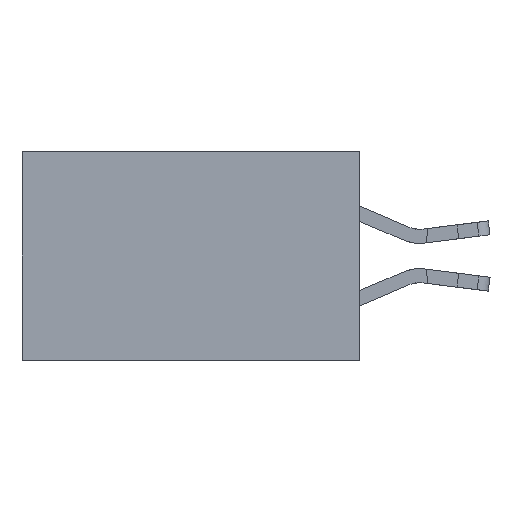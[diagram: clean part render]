
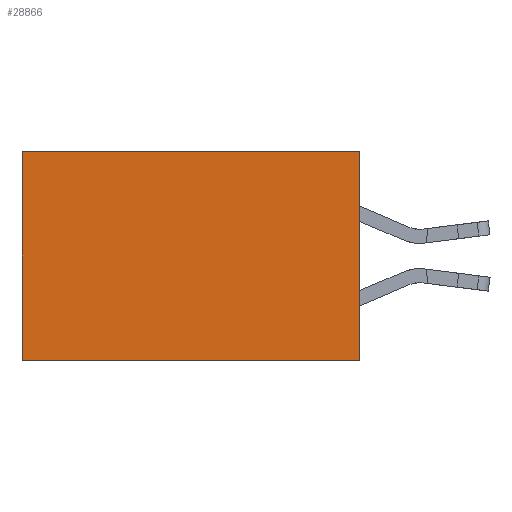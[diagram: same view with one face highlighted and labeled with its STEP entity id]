
A CAD part, left-side view. The second image highlights one B-rep face of the part: STEP entity #28866.
In plain terms, the highlighted planar face has unit normal (-1, 0, 0).
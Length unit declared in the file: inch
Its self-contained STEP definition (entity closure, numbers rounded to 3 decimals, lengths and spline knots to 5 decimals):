
#1132 = PLANE ( 'NONE',  #10331 ) ;
#1287 = CARTESIAN_POINT ( 'NONE',  ( 0.2875, 0., 0. ) ) ;
#1408 = EDGE_CURVE ( 'NONE', #7992, #14091, #3593, .T. ) ;
#1514 = CARTESIAN_POINT ( 'NONE',  ( 0.2875, 0.6, 0. ) ) ;
#1757 = CARTESIAN_POINT ( 'NONE',  ( 0.2875, 0., -0.37 ) ) ;
#1808 = DIRECTION ( 'NONE',  ( 0., 0., -1. ) ) ;
#2328 = LINE ( 'NONE', #1287, #7299 ) ;
#3593 = LINE ( 'NONE', #5527, #18698 ) ;
#3740 = DIRECTION ( 'NONE',  ( 0., 0., -1. ) ) ;
#5527 = CARTESIAN_POINT ( 'NONE',  ( 0.2875, 0., 0. ) ) ;
#5726 = DIRECTION ( 'NONE',  ( 0., 1., 0. ) ) ;
#5927 = ORIENTED_EDGE ( 'NONE', *, *, #18400, .F. ) ;
#7299 = VECTOR ( 'NONE', #3740, 39.37008 ) ;
#7992 = VERTEX_POINT ( 'NONE', #8667 ) ;
#8015 = DIRECTION ( 'NONE',  ( 1., 0., 0. ) ) ;
#8667 = CARTESIAN_POINT ( 'NONE',  ( 0.2875, 0., 0. ) ) ;
#9554 = CARTESIAN_POINT ( 'NONE',  ( 0.2875, 0., -0.37 ) ) ;
#10331 = AXIS2_PLACEMENT_3D ( 'NONE', #26104, #8015, #25819 ) ;
#11469 = EDGE_LOOP ( 'NONE', ( #28283, #20543, #5927, #12987 ) ) ;
#11932 = LINE ( 'NONE', #1514, #24265 ) ;
#12057 = EDGE_CURVE ( 'NONE', #25491, #14859, #18609, .T. ) ;
#12987 = ORIENTED_EDGE ( 'NONE', *, *, #1408, .T. ) ;
#13272 = CARTESIAN_POINT ( 'NONE',  ( 0.2875, 0.6, 0. ) ) ;
#14091 = VERTEX_POINT ( 'NONE', #13272 ) ;
#14859 = VERTEX_POINT ( 'NONE', #18340 ) ;
#15026 = FACE_OUTER_BOUND ( 'NONE', #11469, .T. ) ;
#18340 = CARTESIAN_POINT ( 'NONE',  ( 0.2875, 0.6, -0.37 ) ) ;
#18400 = EDGE_CURVE ( 'NONE', #7992, #25491, #2328, .T. ) ;
#18609 = LINE ( 'NONE', #9554, #20760 ) ;
#18698 = VECTOR ( 'NONE', #5726, 39.37008 ) ;
#20543 = ORIENTED_EDGE ( 'NONE', *, *, #12057, .F. ) ;
#20760 = VECTOR ( 'NONE', #20972, 39.37008 ) ;
#20972 = DIRECTION ( 'NONE',  ( 0., 1., 0. ) ) ;
#24265 = VECTOR ( 'NONE', #1808, 39.37008 ) ;
#25491 = VERTEX_POINT ( 'NONE', #1757 ) ;
#25819 = DIRECTION ( 'NONE',  ( 0., 0., -1. ) ) ;
#26104 = CARTESIAN_POINT ( 'NONE',  ( 0.2875, 0., 0. ) ) ;
#28283 = ORIENTED_EDGE ( 'NONE', *, *, #29047, .T. ) ;
#28866 = ADVANCED_FACE ( 'NONE', ( #15026 ), #1132, .F. ) ;
#29047 = EDGE_CURVE ( 'NONE', #14091, #14859, #11932, .T. ) ;
